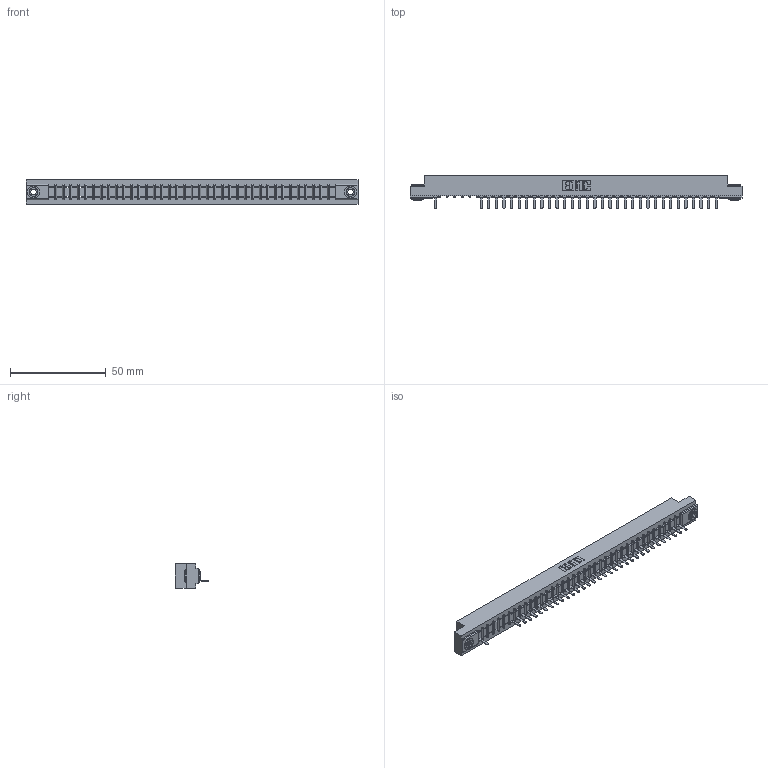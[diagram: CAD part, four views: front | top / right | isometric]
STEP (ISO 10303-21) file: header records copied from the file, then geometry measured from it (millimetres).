
FILE_DESCRIPTION (( 'STEP AP203' ), '1' );
FILE_NAME ('357-038-521-103.STEP', '2018-08-10T09:08:44', ( '' ), ( '' ), 'SwSTEP 2.0', 'SolidWorks 2016', '' );
FILE_SCHEMA (( 'CONFIG_CONTROL_DESIGN' ));
Length unit declared in the file: inch
Products named in the file (4): 357-038-521-103; 307 Part_.156 Dia Mounting Holes; 307-290-002_521; 345-250-002_345-250-002-102
Assembly tree (36 placements, depth 2):
  357-038-521-103
    307 Part_.156 Dia Mounting Holes
    307-290-002_521  x33
    345-250-002_345-250-002-102  x2
Bounding box: 173.58 x 17.42 x 12.7 mm (x, y, z)
Volume: 18404.4 mm3; surface area: 22381.3 mm2
Topology: 36 solids, 36 shells, 2751 faces, 8411 edges, 5498 vertices
Faces by surface type: plane 1639, cylinder 1026, sphere 78, cone 8
Entity records: 34693 total; most frequent: CARTESIAN_POINT 5852, ORIENTED_EDGE 5838, DIRECTION 5697, EDGE_CURVE 2919, LINE 2227, VECTOR 2227, VERTEX_POINT 1890, AXIS2_PLACEMENT_3D 1735
